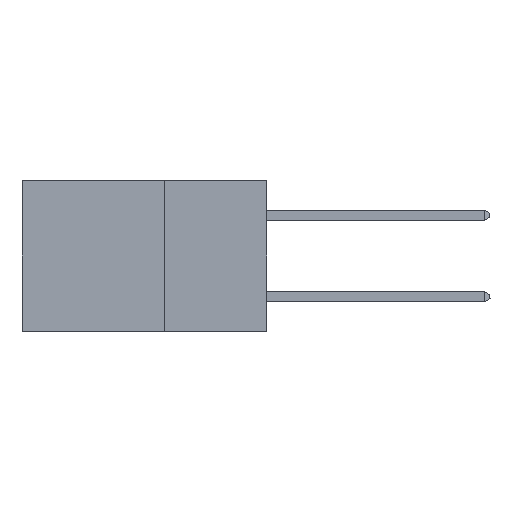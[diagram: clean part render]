
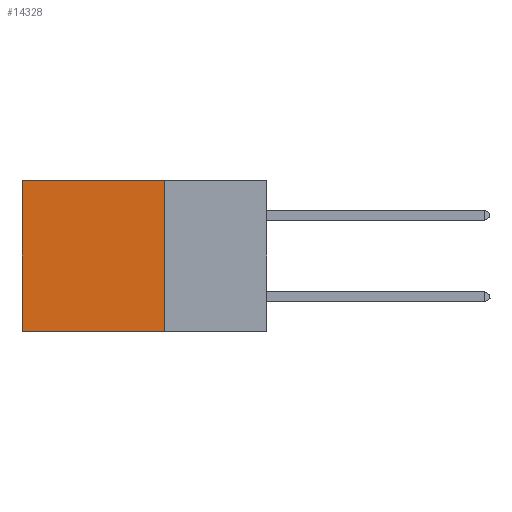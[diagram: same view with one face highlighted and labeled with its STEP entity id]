
A CAD part, left-side view. The second image highlights one B-rep face of the part: STEP entity #14328.
In plain terms, the highlighted planar face has unit normal (-1, 0, 0).
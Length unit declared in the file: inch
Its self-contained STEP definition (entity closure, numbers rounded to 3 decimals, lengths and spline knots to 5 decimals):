
#291 = EDGE_CURVE ( 'NONE', #8679, #483, #16636, .T. ) ;
#369 = VECTOR ( 'NONE', #12238, 39.37008 ) ;
#483 = VERTEX_POINT ( 'NONE', #18486 ) ;
#1555 = LINE ( 'NONE', #1663, #8849 ) ;
#1663 = CARTESIAN_POINT ( 'NONE',  ( 0.2875, 0.6, 0. ) ) ;
#1951 = ORIENTED_EDGE ( 'NONE', *, *, #291, .F. ) ;
#2520 = ORIENTED_EDGE ( 'NONE', *, *, #16448, .T. ) ;
#2854 = CARTESIAN_POINT ( 'NONE',  ( 0.2875, 0.6, -0.37 ) ) ;
#2902 = VERTEX_POINT ( 'NONE', #2854 ) ;
#3393 = ORIENTED_EDGE ( 'NONE', *, *, #15960, .T. ) ;
#3970 = DIRECTION ( 'NONE',  ( 0., 0., -1. ) ) ;
#4228 = VECTOR ( 'NONE', #3970, 39.37008 ) ;
#4603 = CARTESIAN_POINT ( 'NONE',  ( 0.2875, 0.25, -0.37 ) ) ;
#4875 = DIRECTION ( 'NONE',  ( 0., 1., 0. ) ) ;
#6704 = CARTESIAN_POINT ( 'NONE',  ( 0.2875, 0.25, 0. ) ) ;
#7441 = DIRECTION ( 'NONE',  ( 0., 0., -1. ) ) ;
#7975 = FACE_OUTER_BOUND ( 'NONE', #11053, .T. ) ;
#8373 = CARTESIAN_POINT ( 'NONE',  ( 0.2875, 0.25, 0. ) ) ;
#8679 = VERTEX_POINT ( 'NONE', #9567 ) ;
#8849 = VECTOR ( 'NONE', #7441, 39.37008 ) ;
#9026 = CARTESIAN_POINT ( 'NONE',  ( 0.2875, 0.25, 0. ) ) ;
#9567 = CARTESIAN_POINT ( 'NONE',  ( 0.2875, 0.25, 0. ) ) ;
#11026 = ORIENTED_EDGE ( 'NONE', *, *, #11318, .F. ) ;
#11053 = EDGE_LOOP ( 'NONE', ( #2520, #11026, #1951, #3393 ) ) ;
#11318 = EDGE_CURVE ( 'NONE', #483, #2902, #17745, .T. ) ;
#12238 = DIRECTION ( 'NONE',  ( 0., 1., 0. ) ) ;
#13689 = DIRECTION ( 'NONE',  ( 1., 0., 0. ) ) ;
#13748 = PLANE ( 'NONE',  #14351 ) ;
#14328 = ADVANCED_FACE ( 'NONE', ( #7975 ), #13748, .F. ) ;
#14351 = AXIS2_PLACEMENT_3D ( 'NONE', #6704, #13689, #15164 ) ;
#15143 = LINE ( 'NONE', #9026, #18286 ) ;
#15164 = DIRECTION ( 'NONE',  ( 0., 0., -1. ) ) ;
#15556 = CARTESIAN_POINT ( 'NONE',  ( 0.2875, 0.6, 0. ) ) ;
#15960 = EDGE_CURVE ( 'NONE', #8679, #18658, #15143, .T. ) ;
#16448 = EDGE_CURVE ( 'NONE', #18658, #2902, #1555, .T. ) ;
#16636 = LINE ( 'NONE', #8373, #4228 ) ;
#17745 = LINE ( 'NONE', #4603, #369 ) ;
#18286 = VECTOR ( 'NONE', #4875, 39.37008 ) ;
#18486 = CARTESIAN_POINT ( 'NONE',  ( 0.2875, 0.25, -0.37 ) ) ;
#18658 = VERTEX_POINT ( 'NONE', #15556 ) ;
